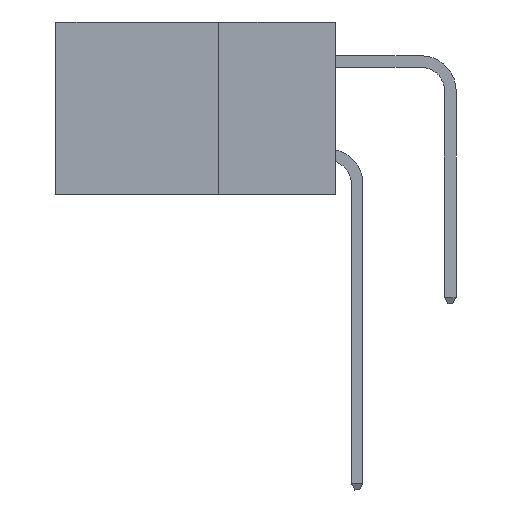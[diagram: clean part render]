
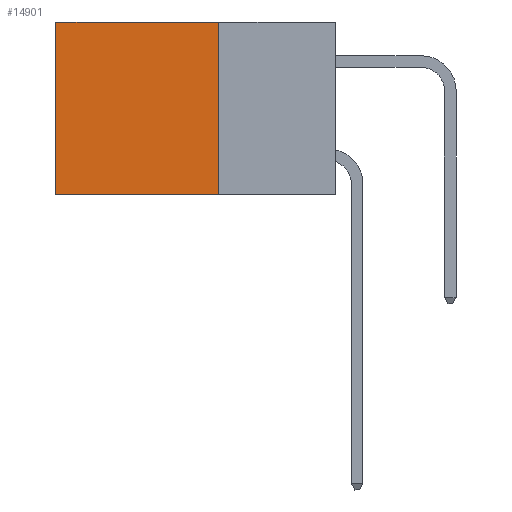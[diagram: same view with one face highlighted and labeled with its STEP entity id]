
A CAD part, left-side view. The second image highlights one B-rep face of the part: STEP entity #14901.
In plain terms, the highlighted planar face has unit normal (-1, 0, 0).
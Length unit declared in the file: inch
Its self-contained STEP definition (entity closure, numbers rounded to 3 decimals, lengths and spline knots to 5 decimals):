
#811 = PLANE ( 'NONE',  #12374 ) ;
#1528 = VECTOR ( 'NONE', #20314, 39.37008 ) ;
#2500 = DIRECTION ( 'NONE',  ( 1., 0., 0. ) ) ;
#2780 = ORIENTED_EDGE ( 'NONE', *, *, #17736, .T. ) ;
#3088 = CARTESIAN_POINT ( 'NONE',  ( 0.2875, 0.6, -0.37 ) ) ;
#4116 = FACE_OUTER_BOUND ( 'NONE', #13680, .T. ) ;
#4290 = VERTEX_POINT ( 'NONE', #9104 ) ;
#4748 = ORIENTED_EDGE ( 'NONE', *, *, #9194, .F. ) ;
#4881 = CARTESIAN_POINT ( 'NONE',  ( 0.2875, 0.6, 0. ) ) ;
#4946 = EDGE_CURVE ( 'NONE', #4290, #19040, #14522, .T. ) ;
#6537 = DIRECTION ( 'NONE',  ( 0., 0., -1. ) ) ;
#8861 = VECTOR ( 'NONE', #6537, 39.37008 ) ;
#9005 = CARTESIAN_POINT ( 'NONE',  ( 0.2875, 0.25, 0. ) ) ;
#9068 = VECTOR ( 'NONE', #20566, 39.37008 ) ;
#9104 = CARTESIAN_POINT ( 'NONE',  ( 0.2875, 0.25, 0. ) ) ;
#9194 = EDGE_CURVE ( 'NONE', #15099, #20272, #19241, .T. ) ;
#10809 = VECTOR ( 'NONE', #15156, 39.37008 ) ;
#11550 = ORIENTED_EDGE ( 'NONE', *, *, #18371, .F. ) ;
#11887 = CARTESIAN_POINT ( 'NONE',  ( 0.2875, 0.25, -0.37 ) ) ;
#12075 = ORIENTED_EDGE ( 'NONE', *, *, #4946, .T. ) ;
#12374 = AXIS2_PLACEMENT_3D ( 'NONE', #9005, #2500, #13865 ) ;
#12652 = CARTESIAN_POINT ( 'NONE',  ( 0.2875, 0.25, 0. ) ) ;
#13348 = LINE ( 'NONE', #12652, #9068 ) ;
#13680 = EDGE_LOOP ( 'NONE', ( #2780, #4748, #11550, #12075 ) ) ;
#13865 = DIRECTION ( 'NONE',  ( 0., 0., -1. ) ) ;
#14155 = LINE ( 'NONE', #4881, #8861 ) ;
#14331 = CARTESIAN_POINT ( 'NONE',  ( 0.2875, 0.6, 0. ) ) ;
#14522 = LINE ( 'NONE', #18774, #1528 ) ;
#14901 = ADVANCED_FACE ( 'NONE', ( #4116 ), #811, .F. ) ;
#15099 = VERTEX_POINT ( 'NONE', #19294 ) ;
#15156 = DIRECTION ( 'NONE',  ( 0., 1., 0. ) ) ;
#17736 = EDGE_CURVE ( 'NONE', #19040, #20272, #14155, .T. ) ;
#18371 = EDGE_CURVE ( 'NONE', #4290, #15099, #13348, .T. ) ;
#18774 = CARTESIAN_POINT ( 'NONE',  ( 0.2875, 0.25, 0. ) ) ;
#19040 = VERTEX_POINT ( 'NONE', #14331 ) ;
#19241 = LINE ( 'NONE', #11887, #10809 ) ;
#19294 = CARTESIAN_POINT ( 'NONE',  ( 0.2875, 0.25, -0.37 ) ) ;
#20272 = VERTEX_POINT ( 'NONE', #3088 ) ;
#20314 = DIRECTION ( 'NONE',  ( 0., 1., 0. ) ) ;
#20566 = DIRECTION ( 'NONE',  ( 0., 0., -1. ) ) ;
